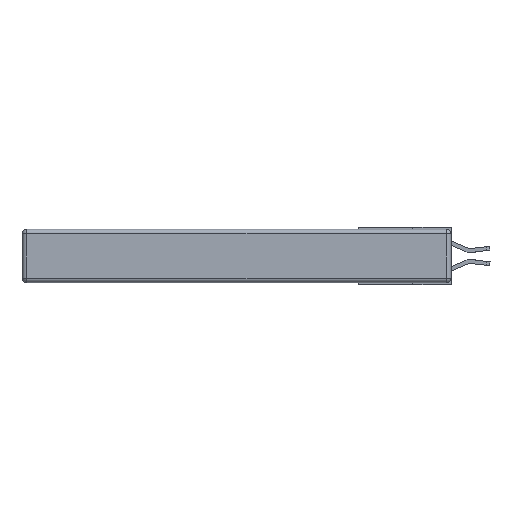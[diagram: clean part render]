
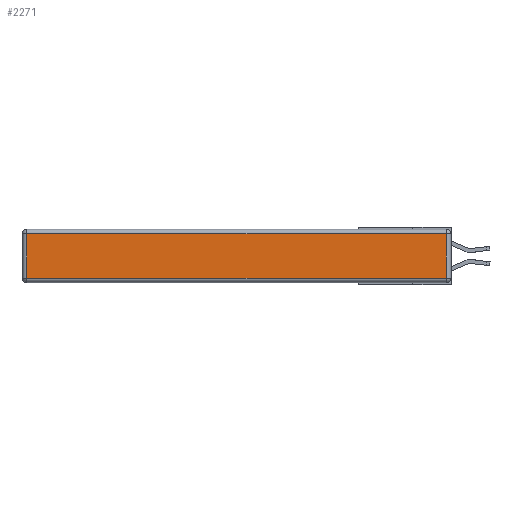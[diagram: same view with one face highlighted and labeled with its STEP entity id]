
A CAD part, left-side view. The second image highlights one B-rep face of the part: STEP entity #2271.
In plain terms, the highlighted planar face has unit normal (-1, 0, 0).
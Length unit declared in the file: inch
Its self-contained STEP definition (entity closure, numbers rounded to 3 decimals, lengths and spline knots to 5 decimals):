
#303 = VERTEX_POINT ( 'NONE', #11703 ) ;
#439 = CARTESIAN_POINT ( 'NONE',  ( 0., 2.72, -0.03 ) ) ;
#974 = CARTESIAN_POINT ( 'NONE',  ( 0., 0., -0.313 ) ) ;
#1524 = DIRECTION ( 'NONE',  ( 0., 1., 0. ) ) ;
#1668 = LINE ( 'NONE', #10899, #4678 ) ;
#1784 = DIRECTION ( 'NONE',  ( 0., 0., 1. ) ) ;
#2115 = ORIENTED_EDGE ( 'NONE', *, *, #5733, .T. ) ;
#2149 = AXIS2_PLACEMENT_3D ( 'NONE', #10947, #6928, #1784 ) ;
#2271 = ADVANCED_FACE ( 'NONE', ( #5037 ), #11042, .T. ) ;
#2824 = ORIENTED_EDGE ( 'NONE', *, *, #6861, .T. ) ;
#3638 = DIRECTION ( 'NONE',  ( 0., 0., -1. ) ) ;
#4678 = VECTOR ( 'NONE', #3638, 39.37008 ) ;
#4727 = CARTESIAN_POINT ( 'NONE',  ( 0., 0.03, -0.343 ) ) ;
#4800 = VECTOR ( 'NONE', #8646, 39.37008 ) ;
#5037 = FACE_OUTER_BOUND ( 'NONE', #10551, .T. ) ;
#5527 = VERTEX_POINT ( 'NONE', #439 ) ;
#5733 = EDGE_CURVE ( 'NONE', #5527, #5798, #1668, .T. ) ;
#5778 = VECTOR ( 'NONE', #10173, 39.37008 ) ;
#5798 = VERTEX_POINT ( 'NONE', #5817 ) ;
#5817 = CARTESIAN_POINT ( 'NONE',  ( 0., 2.72, -0.313 ) ) ;
#6529 = ORIENTED_EDGE ( 'NONE', *, *, #8884, .T. ) ;
#6861 = EDGE_CURVE ( 'NONE', #5798, #303, #7521, .T. ) ;
#6928 = DIRECTION ( 'NONE',  ( -1., 0., 0. ) ) ;
#7147 = EDGE_CURVE ( 'NONE', #12879, #5527, #8990, .T. ) ;
#7521 = LINE ( 'NONE', #974, #5778 ) ;
#7648 = CARTESIAN_POINT ( 'NONE',  ( 0., 2.75, -0.03 ) ) ;
#7720 = ORIENTED_EDGE ( 'NONE', *, *, #7147, .T. ) ;
#8646 = DIRECTION ( 'NONE',  ( 0., 0., 1. ) ) ;
#8884 = EDGE_CURVE ( 'NONE', #303, #12879, #9082, .T. ) ;
#8990 = LINE ( 'NONE', #7648, #11350 ) ;
#9082 = LINE ( 'NONE', #4727, #4800 ) ;
#10173 = DIRECTION ( 'NONE',  ( 0., -1., 0. ) ) ;
#10445 = CARTESIAN_POINT ( 'NONE',  ( 0., 0.03, -0.03 ) ) ;
#10551 = EDGE_LOOP ( 'NONE', ( #2824, #6529, #7720, #2115 ) ) ;
#10899 = CARTESIAN_POINT ( 'NONE',  ( 0., 2.72, -0.343 ) ) ;
#10947 = CARTESIAN_POINT ( 'NONE',  ( 0., 0., -0.343 ) ) ;
#11042 = PLANE ( 'NONE',  #2149 ) ;
#11350 = VECTOR ( 'NONE', #1524, 39.37008 ) ;
#11703 = CARTESIAN_POINT ( 'NONE',  ( 0., 0.03, -0.313 ) ) ;
#12879 = VERTEX_POINT ( 'NONE', #10445 ) ;
